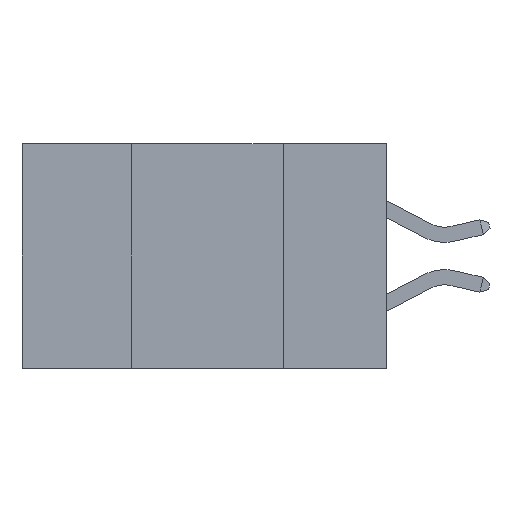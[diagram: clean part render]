
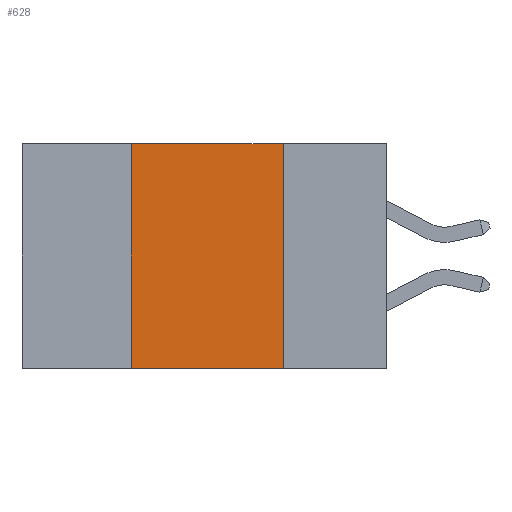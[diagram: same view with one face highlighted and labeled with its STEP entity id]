
A CAD part, left-side view. The second image highlights one B-rep face of the part: STEP entity #628.
In plain terms, the highlighted planar face has unit normal (-1, 0, 0).
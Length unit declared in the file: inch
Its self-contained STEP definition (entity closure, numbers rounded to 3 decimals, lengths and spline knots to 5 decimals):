
#628 = ADVANCED_FACE ( 'NONE', ( #10580 ), #12640, .F. ) ;
#686 = CARTESIAN_POINT ( 'NONE',  ( 0., 0.6, 0. ) ) ;
#910 = DIRECTION ( 'NONE',  ( 0., 0., -1. ) ) ;
#1058 = ORIENTED_EDGE ( 'NONE', *, *, #3101, .F. ) ;
#1988 = VERTEX_POINT ( 'NONE', #3191 ) ;
#2198 = CARTESIAN_POINT ( 'NONE',  ( 0., 0.17, 0. ) ) ;
#2366 = CARTESIAN_POINT ( 'NONE',  ( 0., 0.42, 0. ) ) ;
#2760 = LINE ( 'NONE', #2366, #7951 ) ;
#2999 = CARTESIAN_POINT ( 'NONE',  ( 0., 0.17, -0.37 ) ) ;
#3082 = LINE ( 'NONE', #686, #8277 ) ;
#3089 = CARTESIAN_POINT ( 'NONE',  ( 0., 0.17, 0. ) ) ;
#3101 = EDGE_CURVE ( 'NONE', #1988, #5658, #3082, .T. ) ;
#3191 = CARTESIAN_POINT ( 'NONE',  ( 0., 0.42, 0. ) ) ;
#3221 = AXIS2_PLACEMENT_3D ( 'NONE', #12320, #3317, #910 ) ;
#3317 = DIRECTION ( 'NONE',  ( 1., 0., 0. ) ) ;
#4003 = DIRECTION ( 'NONE',  ( 0., -1., 0. ) ) ;
#4471 = DIRECTION ( 'NONE',  ( 0., 0., 1. ) ) ;
#5029 = CARTESIAN_POINT ( 'NONE',  ( 0., 0.6, -0.37 ) ) ;
#5112 = CARTESIAN_POINT ( 'NONE',  ( 0., 0.42, -0.37 ) ) ;
#5254 = EDGE_LOOP ( 'NONE', ( #10383, #1058, #8915, #13080 ) ) ;
#5658 = VERTEX_POINT ( 'NONE', #3089 ) ;
#6375 = DIRECTION ( 'NONE',  ( 0., 0., -1. ) ) ;
#6467 = EDGE_CURVE ( 'NONE', #5658, #9410, #12365, .T. ) ;
#7951 = VECTOR ( 'NONE', #4471, 39.37008 ) ;
#8137 = EDGE_CURVE ( 'NONE', #12582, #9410, #12957, .T. ) ;
#8277 = VECTOR ( 'NONE', #10178, 39.37008 ) ;
#8915 = ORIENTED_EDGE ( 'NONE', *, *, #9640, .F. ) ;
#9410 = VERTEX_POINT ( 'NONE', #2999 ) ;
#9640 = EDGE_CURVE ( 'NONE', #12582, #1988, #2760, .T. ) ;
#9674 = VECTOR ( 'NONE', #6375, 39.37008 ) ;
#10178 = DIRECTION ( 'NONE',  ( 0., -1., 0. ) ) ;
#10383 = ORIENTED_EDGE ( 'NONE', *, *, #6467, .F. ) ;
#10580 = FACE_OUTER_BOUND ( 'NONE', #5254, .T. ) ;
#12320 = CARTESIAN_POINT ( 'NONE',  ( 0., 0.6, 0. ) ) ;
#12365 = LINE ( 'NONE', #2198, #9674 ) ;
#12582 = VERTEX_POINT ( 'NONE', #5112 ) ;
#12640 = PLANE ( 'NONE',  #3221 ) ;
#12646 = VECTOR ( 'NONE', #4003, 39.37008 ) ;
#12957 = LINE ( 'NONE', #5029, #12646 ) ;
#13080 = ORIENTED_EDGE ( 'NONE', *, *, #8137, .T. ) ;
